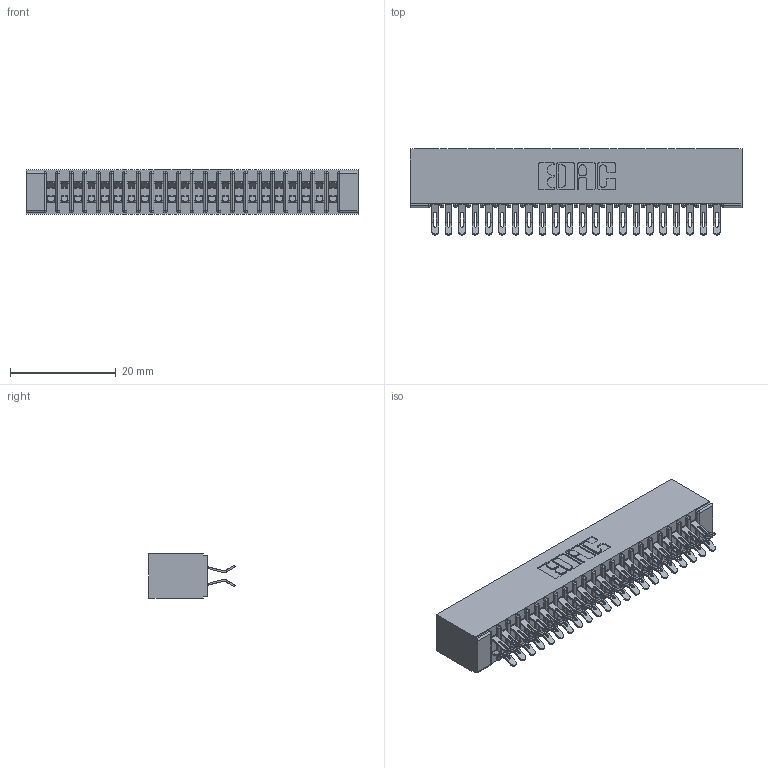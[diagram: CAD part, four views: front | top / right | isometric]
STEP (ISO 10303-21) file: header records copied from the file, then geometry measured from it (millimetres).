
FILE_DESCRIPTION (( 'STEP AP203' ), '1' );
FILE_NAME ('341-044-555-201.STEP', '2018-08-07T02:42:03', ( '' ), ( '' ), 'SwSTEP 2.0', 'SolidWorks 2016', '' );
FILE_SCHEMA (( 'CONFIG_CONTROL_DESIGN' ));
Length unit declared in the file: inch
Products named in the file (3): 341 Part_No Mounting Lugs; 341-292-001_341-292-155; 341-044-555-201
Assembly tree (45 placements, depth 2):
  341-044-555-201
    341 Part_No Mounting Lugs
    341-292-001_341-292-155  x44
Bounding box: 62.87 x 16.31 x 8.38 mm (x, y, z)
Volume: 3763.7 mm3; surface area: 8856.9 mm2
Topology: 45 solids, 45 shells, 3540 faces, 10566 edges, 6878 vertices
Faces by surface type: plane 1912, cylinder 1540, sphere 46, torus 42
Entity records: 29481 total; most frequent: CARTESIAN_POINT 4916, ORIENTED_EDGE 4872, DIRECTION 4774, EDGE_CURVE 2436, LINE 1934, VECTOR 1934, VERTEX_POINT 1546, AXIS2_PLACEMENT_3D 1420
